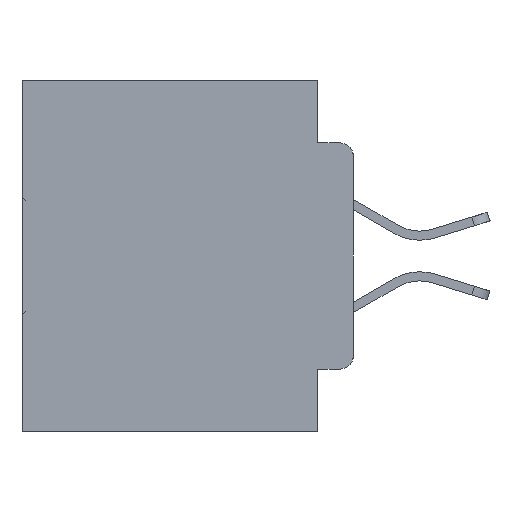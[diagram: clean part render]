
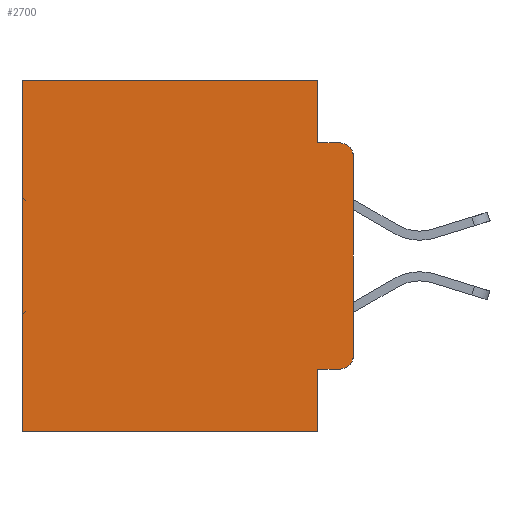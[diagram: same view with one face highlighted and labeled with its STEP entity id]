
A CAD part, left-side view. The second image highlights one B-rep face of the part: STEP entity #2700.
In plain terms, the highlighted planar face has unit normal (-1, 0, 0).
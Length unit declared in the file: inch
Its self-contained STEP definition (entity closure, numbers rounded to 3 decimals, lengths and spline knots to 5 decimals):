
#846 = CARTESIAN_POINT ( 'NONE',  ( 0.298, 0., 0. ) ) ;
#1294 = EDGE_CURVE ( 'NONE', #21294, #8213, #13464, .T. ) ;
#1571 = VECTOR ( 'NONE', #31460, 39.37008 ) ;
#2700 = ADVANCED_FACE ( 'NONE', ( #28764 ), #5071, .F. ) ;
#3060 = EDGE_CURVE ( 'NONE', #8213, #23747, #23954, .T. ) ;
#3104 = CARTESIAN_POINT ( 'NONE',  ( 0.298, 0.473, 0. ) ) ;
#3254 = CARTESIAN_POINT ( 'NONE',  ( 0.298, 0.02, -0.3915 ) ) ;
#3625 = ORIENTED_EDGE ( 'NONE', *, *, #4855, .T. ) ;
#4044 = ORIENTED_EDGE ( 'NONE', *, *, #29928, .T. ) ;
#4180 = VERTEX_POINT ( 'NONE', #6718 ) ;
#4855 = EDGE_CURVE ( 'NONE', #25824, #23747, #33043, .T. ) ;
#5071 = PLANE ( 'NONE',  #26283 ) ;
#5186 = LINE ( 'NONE', #9779, #18298 ) ;
#5228 = DIRECTION ( 'NONE',  ( 0., 0., -1. ) ) ;
#5920 = DIRECTION ( 'NONE',  ( 0., 0., -1. ) ) ;
#6272 = CIRCLE ( 'NONE', #24629, 0.02 ) ;
#6371 = VERTEX_POINT ( 'NONE', #10720 ) ;
#6470 = VECTOR ( 'NONE', #32868, 39.37008 ) ;
#6718 = CARTESIAN_POINT ( 'NONE',  ( 0.298, 0., -0.3915 ) ) ;
#6838 = CARTESIAN_POINT ( 'NONE',  ( 0.298, 0., 0. ) ) ;
#8120 = CARTESIAN_POINT ( 'NONE',  ( 0.298, 0., -0.1085 ) ) ;
#8213 = VERTEX_POINT ( 'NONE', #12997 ) ;
#8736 = DIRECTION ( 'NONE',  ( 0., 1., 0. ) ) ;
#9105 = CARTESIAN_POINT ( 'NONE',  ( 0.298, 0., -0.5 ) ) ;
#9141 = LINE ( 'NONE', #24083, #22229 ) ;
#9220 = DIRECTION ( 'NONE',  ( 1., 0., 0. ) ) ;
#9384 = ORIENTED_EDGE ( 'NONE', *, *, #16769, .T. ) ;
#9410 = LINE ( 'NONE', #21244, #1571 ) ;
#9779 = CARTESIAN_POINT ( 'NONE',  ( 0.298, 0.473, 0. ) ) ;
#10464 = VECTOR ( 'NONE', #20077, 39.37008 ) ;
#10720 = CARTESIAN_POINT ( 'NONE',  ( 0.298, 0.473, -0.5 ) ) ;
#11933 = EDGE_CURVE ( 'NONE', #25824, #4180, #16156, .T. ) ;
#12805 = VECTOR ( 'NONE', #8736, 39.37008 ) ;
#12997 = CARTESIAN_POINT ( 'NONE',  ( 0.298, 0.051, -0.0885 ) ) ;
#13090 = AXIS2_PLACEMENT_3D ( 'NONE', #30093, #18092, #18039 ) ;
#13464 = LINE ( 'NONE', #32186, #6470 ) ;
#14366 = ORIENTED_EDGE ( 'NONE', *, *, #26480, .F. ) ;
#14753 = ORIENTED_EDGE ( 'NONE', *, *, #1294, .F. ) ;
#16060 = EDGE_CURVE ( 'NONE', #32928, #4180, #6272, .T. ) ;
#16156 = LINE ( 'NONE', #6838, #29117 ) ;
#16165 = VERTEX_POINT ( 'NONE', #19311 ) ;
#16614 = CARTESIAN_POINT ( 'NONE',  ( 0.298, 0.051, 0. ) ) ;
#16769 = EDGE_CURVE ( 'NONE', #21294, #22796, #33387, .T. ) ;
#17801 = EDGE_CURVE ( 'NONE', #16165, #32928, #9410, .T. ) ;
#17865 = CARTESIAN_POINT ( 'NONE',  ( 0.298, 0.02, -0.0885 ) ) ;
#17905 = VECTOR ( 'NONE', #19522, 39.37008 ) ;
#18039 = DIRECTION ( 'NONE',  ( 0., 0., -1. ) ) ;
#18092 = DIRECTION ( 'NONE',  ( -1., 0., 0. ) ) ;
#18298 = VECTOR ( 'NONE', #25495, 39.37008 ) ;
#19311 = CARTESIAN_POINT ( 'NONE',  ( 0.298, 0.051, -0.4115 ) ) ;
#19522 = DIRECTION ( 'NONE',  ( 0., 1., 0. ) ) ;
#20077 = DIRECTION ( 'NONE',  ( 0., -1., 0. ) ) ;
#20117 = CARTESIAN_POINT ( 'NONE',  ( 0.298, 0.051, -0.0885 ) ) ;
#21244 = CARTESIAN_POINT ( 'NONE',  ( 0.298, 0.051, -0.4115 ) ) ;
#21294 = VERTEX_POINT ( 'NONE', #16614 ) ;
#21591 = DIRECTION ( 'NONE',  ( -1., 0., 0. ) ) ;
#22229 = VECTOR ( 'NONE', #26657, 39.37008 ) ;
#22705 = EDGE_LOOP ( 'NONE', ( #28904, #3625, #32875, #14753, #9384, #4044, #25700, #14366, #22882, #31296 ) ) ;
#22796 = VERTEX_POINT ( 'NONE', #3104 ) ;
#22882 = ORIENTED_EDGE ( 'NONE', *, *, #17801, .T. ) ;
#23747 = VERTEX_POINT ( 'NONE', #17865 ) ;
#23954 = LINE ( 'NONE', #20117, #10464 ) ;
#24083 = CARTESIAN_POINT ( 'NONE',  ( 0.298, 0.051, 0. ) ) ;
#24629 = AXIS2_PLACEMENT_3D ( 'NONE', #3254, #21591, #5920 ) ;
#25495 = DIRECTION ( 'NONE',  ( 0., 0., -1. ) ) ;
#25700 = ORIENTED_EDGE ( 'NONE', *, *, #29733, .F. ) ;
#25824 = VERTEX_POINT ( 'NONE', #8120 ) ;
#26283 = AXIS2_PLACEMENT_3D ( 'NONE', #846, #9220, #5228 ) ;
#26480 = EDGE_CURVE ( 'NONE', #16165, #28380, #9141, .T. ) ;
#26657 = DIRECTION ( 'NONE',  ( 0., 0., -1. ) ) ;
#26951 = CARTESIAN_POINT ( 'NONE',  ( 0.298, 0., 0. ) ) ;
#27656 = DIRECTION ( 'NONE',  ( 0., 0., -1. ) ) ;
#28380 = VERTEX_POINT ( 'NONE', #31624 ) ;
#28764 = FACE_OUTER_BOUND ( 'NONE', #22705, .T. ) ;
#28904 = ORIENTED_EDGE ( 'NONE', *, *, #11933, .F. ) ;
#29117 = VECTOR ( 'NONE', #27656, 39.37008 ) ;
#29733 = EDGE_CURVE ( 'NONE', #28380, #6371, #31602, .T. ) ;
#29928 = EDGE_CURVE ( 'NONE', #22796, #6371, #5186, .T. ) ;
#30093 = CARTESIAN_POINT ( 'NONE',  ( 0.298, 0.02, -0.1085 ) ) ;
#31296 = ORIENTED_EDGE ( 'NONE', *, *, #16060, .T. ) ;
#31460 = DIRECTION ( 'NONE',  ( 0., -1., 0. ) ) ;
#31602 = LINE ( 'NONE', #9105, #17905 ) ;
#31624 = CARTESIAN_POINT ( 'NONE',  ( 0.298, 0.051, -0.5 ) ) ;
#32186 = CARTESIAN_POINT ( 'NONE',  ( 0.298, 0.051, 0. ) ) ;
#32332 = CARTESIAN_POINT ( 'NONE',  ( 0.298, 0.02, -0.4115 ) ) ;
#32868 = DIRECTION ( 'NONE',  ( 0., 0., -1. ) ) ;
#32875 = ORIENTED_EDGE ( 'NONE', *, *, #3060, .F. ) ;
#32928 = VERTEX_POINT ( 'NONE', #32332 ) ;
#33043 = CIRCLE ( 'NONE', #13090, 0.02 ) ;
#33387 = LINE ( 'NONE', #26951, #12805 ) ;
